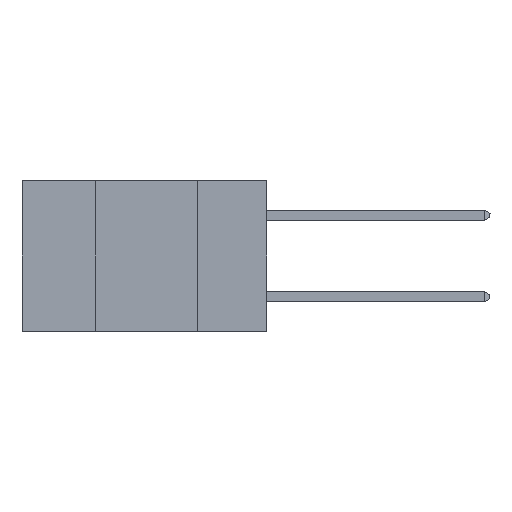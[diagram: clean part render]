
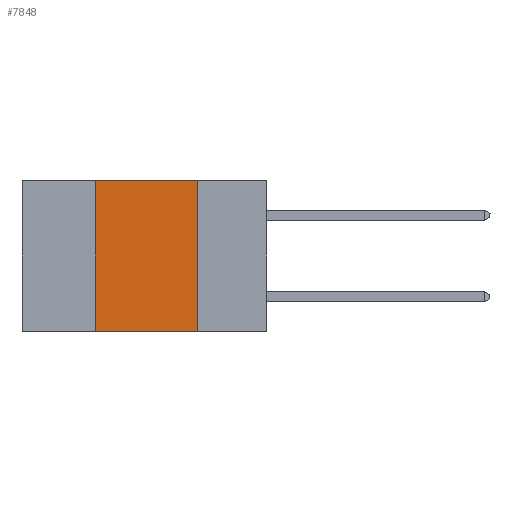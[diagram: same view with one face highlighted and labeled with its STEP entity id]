
A CAD part, left-side view. The second image highlights one B-rep face of the part: STEP entity #7848.
In plain terms, the highlighted planar face has unit normal (-1, 0, 0).
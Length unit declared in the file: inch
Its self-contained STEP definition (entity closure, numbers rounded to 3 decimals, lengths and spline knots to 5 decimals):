
#90 = ORIENTED_EDGE ( 'NONE', *, *, #662, .F. ) ;
#262 = CARTESIAN_POINT ( 'NONE',  ( 0., 0.6, -0.37 ) ) ;
#549 = CARTESIAN_POINT ( 'NONE',  ( 0., 0.42, 0. ) ) ;
#662 = EDGE_CURVE ( 'NONE', #6636, #7784, #2073, .T. ) ;
#1039 = ORIENTED_EDGE ( 'NONE', *, *, #8487, .F. ) ;
#1068 = DIRECTION ( 'NONE',  ( 0., -1., 0. ) ) ;
#1218 = LINE ( 'NONE', #3514, #7871 ) ;
#1360 = CARTESIAN_POINT ( 'NONE',  ( 0., 0.17, -0.37 ) ) ;
#1917 = CARTESIAN_POINT ( 'NONE',  ( 0., 0.42, 0. ) ) ;
#1979 = CARTESIAN_POINT ( 'NONE',  ( 0., 0.6, 0. ) ) ;
#2073 = LINE ( 'NONE', #549, #2811 ) ;
#2266 = EDGE_CURVE ( 'NONE', #7709, #3911, #1218, .T. ) ;
#2811 = VECTOR ( 'NONE', #3775, 39.37008 ) ;
#2813 = CARTESIAN_POINT ( 'NONE',  ( 0., 0.6, 0. ) ) ;
#2915 = PLANE ( 'NONE',  #7824 ) ;
#3489 = ORIENTED_EDGE ( 'NONE', *, *, #2266, .F. ) ;
#3514 = CARTESIAN_POINT ( 'NONE',  ( 0., 0.17, 0. ) ) ;
#3775 = DIRECTION ( 'NONE',  ( 0., 0., 1. ) ) ;
#3911 = VERTEX_POINT ( 'NONE', #1360 ) ;
#3915 = ORIENTED_EDGE ( 'NONE', *, *, #9726, .T. ) ;
#4321 = CARTESIAN_POINT ( 'NONE',  ( 0., 0.17, 0. ) ) ;
#5808 = DIRECTION ( 'NONE',  ( 0., 0., -1. ) ) ;
#6116 = FACE_OUTER_BOUND ( 'NONE', #6677, .T. ) ;
#6636 = VERTEX_POINT ( 'NONE', #6908 ) ;
#6677 = EDGE_LOOP ( 'NONE', ( #3489, #1039, #90, #3915 ) ) ;
#6739 = DIRECTION ( 'NONE',  ( 1., 0., 0. ) ) ;
#6908 = CARTESIAN_POINT ( 'NONE',  ( 0., 0.42, -0.37 ) ) ;
#6963 = DIRECTION ( 'NONE',  ( 0., -1., 0. ) ) ;
#7101 = LINE ( 'NONE', #262, #9379 ) ;
#7709 = VERTEX_POINT ( 'NONE', #4321 ) ;
#7784 = VERTEX_POINT ( 'NONE', #1917 ) ;
#7824 = AXIS2_PLACEMENT_3D ( 'NONE', #1979, #6739, #10028 ) ;
#7848 = ADVANCED_FACE ( 'NONE', ( #6116 ), #2915, .F. ) ;
#7871 = VECTOR ( 'NONE', #5808, 39.37008 ) ;
#8487 = EDGE_CURVE ( 'NONE', #7784, #7709, #10225, .T. ) ;
#8854 = VECTOR ( 'NONE', #6963, 39.37008 ) ;
#9379 = VECTOR ( 'NONE', #1068, 39.37008 ) ;
#9726 = EDGE_CURVE ( 'NONE', #6636, #3911, #7101, .T. ) ;
#10028 = DIRECTION ( 'NONE',  ( 0., 0., -1. ) ) ;
#10225 = LINE ( 'NONE', #2813, #8854 ) ;
